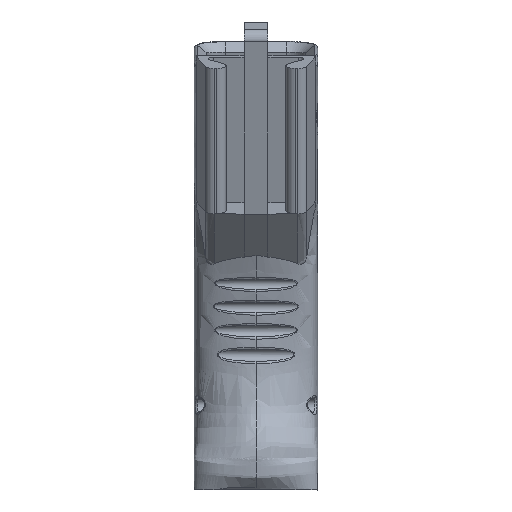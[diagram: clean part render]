
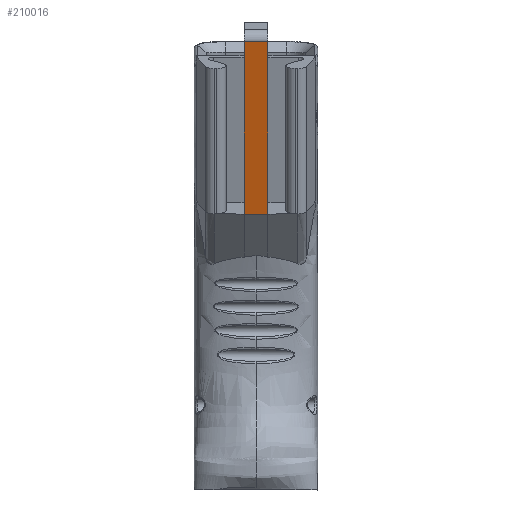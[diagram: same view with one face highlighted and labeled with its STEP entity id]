
A CAD part, left-side view. The second image highlights one B-rep face of the part: STEP entity #210016.
In plain terms, the highlighted planar face has unit normal (-0.951, 0, -0.309).
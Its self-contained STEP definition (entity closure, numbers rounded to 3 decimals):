
#12224 = CARTESIAN_POINT ( 'NONE',  ( 10.35, -2.5, -4.957 ) ) ;
#14920 = DIRECTION ( 'NONE',  ( 0.309, 0., -0.951 ) ) ;
#17638 = VERTEX_POINT ( 'NONE', #21460 ) ;
#21453 = EDGE_CURVE ( 'NONE', #50525, #136074, #28211, .T. ) ;
#21460 = CARTESIAN_POINT ( 'NONE',  ( 10.35, -2.5, -4.957 ) ) ;
#23556 = LINE ( 'NONE', #12224, #42178 ) ;
#28211 = LINE ( 'NONE', #104700, #33379 ) ;
#30692 = CARTESIAN_POINT ( 'NONE',  ( 9.732, -2.5, -3.055 ) ) ;
#33379 = VECTOR ( 'NONE', #84591, 1000. ) ;
#42178 = VECTOR ( 'NONE', #48732, 1000. ) ;
#44914 = ORIENTED_EDGE ( 'NONE', *, *, #21453, .T. ) ;
#45201 = CARTESIAN_POINT ( 'NONE',  ( 22.093, -2.5, -41.097 ) ) ;
#48732 = DIRECTION ( 'NONE',  ( 0., 1., 0. ) ) ;
#49215 = CARTESIAN_POINT ( 'NONE',  ( 9.732, -2.5, -3.055 ) ) ;
#50195 = LINE ( 'NONE', #45201, #73865 ) ;
#50525 = VERTEX_POINT ( 'NONE', #195548 ) ;
#51236 = ORIENTED_EDGE ( 'NONE', *, *, #117244, .T. ) ;
#60467 = CARTESIAN_POINT ( 'NONE',  ( 22.093, -2.5, -41.097 ) ) ;
#63169 = EDGE_LOOP ( 'NONE', ( #220444, #101320, #44914, #51236 ) ) ;
#73865 = VECTOR ( 'NONE', #199019, 1000. ) ;
#84591 = DIRECTION ( 'NONE',  ( 0.309, 0., -0.951 ) ) ;
#89720 = EDGE_CURVE ( 'NONE', #17638, #50525, #23556, .T. ) ;
#101320 = ORIENTED_EDGE ( 'NONE', *, *, #89720, .T. ) ;
#104700 = CARTESIAN_POINT ( 'NONE',  ( 9.732, 2.5, -3.055 ) ) ;
#109706 = VECTOR ( 'NONE', #14920, 1000. ) ;
#117244 = EDGE_CURVE ( 'NONE', #136074, #212125, #50195, .T. ) ;
#119694 = AXIS2_PLACEMENT_3D ( 'NONE', #30692, #217395, #132129 ) ;
#125737 = LINE ( 'NONE', #49215, #109706 ) ;
#128125 = CARTESIAN_POINT ( 'NONE',  ( 22.093, 2.5, -41.097 ) ) ;
#132129 = DIRECTION ( 'NONE',  ( 0.309, 0., -0.951 ) ) ;
#136074 = VERTEX_POINT ( 'NONE', #128125 ) ;
#146298 = FACE_OUTER_BOUND ( 'NONE', #63169, .T. ) ;
#195548 = CARTESIAN_POINT ( 'NONE',  ( 10.35, 2.5, -4.957 ) ) ;
#199019 = DIRECTION ( 'NONE',  ( 0., -1., 0. ) ) ;
#203145 = PLANE ( 'NONE',  #119694 ) ;
#206336 = EDGE_CURVE ( 'NONE', #17638, #212125, #125737, .T. ) ;
#210016 = ADVANCED_FACE ( 'NONE', ( #146298 ), #203145, .F. ) ;
#212125 = VERTEX_POINT ( 'NONE', #60467 ) ;
#217395 = DIRECTION ( 'NONE',  ( 0.951, 0., 0.309 ) ) ;
#220444 = ORIENTED_EDGE ( 'NONE', *, *, #206336, .F. ) ;
